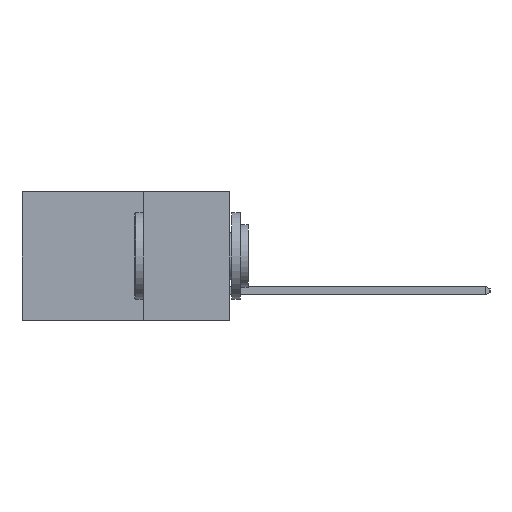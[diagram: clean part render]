
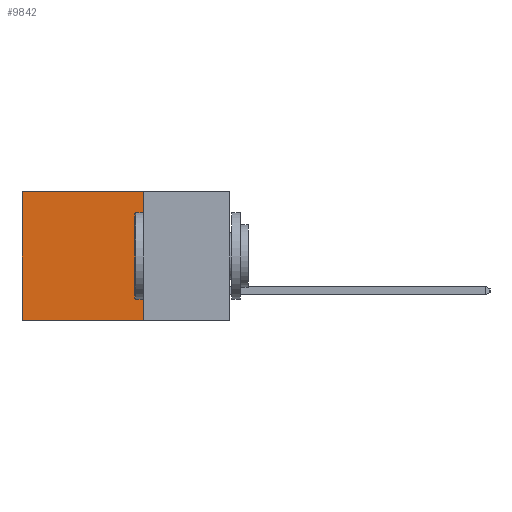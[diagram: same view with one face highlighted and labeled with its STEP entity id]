
A CAD part, left-side view. The second image highlights one B-rep face of the part: STEP entity #9842.
In plain terms, the highlighted planar face has unit normal (-1, 0, 0).
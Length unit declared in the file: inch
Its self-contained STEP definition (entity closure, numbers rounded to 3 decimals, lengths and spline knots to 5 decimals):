
#612 = EDGE_CURVE ( 'NONE', #9151, #3055, #3788, .T. ) ;
#982 = ORIENTED_EDGE ( 'NONE', *, *, #3374, .T. ) ;
#1239 = ORIENTED_EDGE ( 'NONE', *, *, #1735, .F. ) ;
#1649 = VECTOR ( 'NONE', #13019, 39.37008 ) ;
#1735 = EDGE_CURVE ( 'NONE', #12136, #3055, #7342, .T. ) ;
#2565 = CARTESIAN_POINT ( 'NONE',  ( 0.2615, 0.25, 0. ) ) ;
#3055 = VERTEX_POINT ( 'NONE', #4842 ) ;
#3374 = EDGE_CURVE ( 'NONE', #3661, #9151, #10922, .T. ) ;
#3661 = VERTEX_POINT ( 'NONE', #2565 ) ;
#3788 = LINE ( 'NONE', #11688, #6868 ) ;
#4416 = VECTOR ( 'NONE', #4444, 39.37008 ) ;
#4444 = DIRECTION ( 'NONE',  ( 0., 1., 0. ) ) ;
#4549 = VECTOR ( 'NONE', #10312, 39.37008 ) ;
#4842 = CARTESIAN_POINT ( 'NONE',  ( 0.2615, 0.6, -0.37 ) ) ;
#5397 = DIRECTION ( 'NONE',  ( 1., 0., 0. ) ) ;
#5766 = CARTESIAN_POINT ( 'NONE',  ( 0.2615, 0.25, -0.37 ) ) ;
#6208 = CARTESIAN_POINT ( 'NONE',  ( 0.2615, 0.25, -0.37 ) ) ;
#6597 = CARTESIAN_POINT ( 'NONE',  ( 0.2615, 0.25, -0.37 ) ) ;
#6868 = VECTOR ( 'NONE', #7545, 39.37008 ) ;
#7025 = CARTESIAN_POINT ( 'NONE',  ( 0.2615, 0.25, -0.37 ) ) ;
#7342 = LINE ( 'NONE', #6208, #4416 ) ;
#7545 = DIRECTION ( 'NONE',  ( 0., 0., -1. ) ) ;
#7558 = DIRECTION ( 'NONE',  ( 0., 0., -1. ) ) ;
#7623 = FACE_OUTER_BOUND ( 'NONE', #13405, .T. ) ;
#8495 = CARTESIAN_POINT ( 'NONE',  ( 0.2615, 0.25, 0. ) ) ;
#9014 = CARTESIAN_POINT ( 'NONE',  ( 0.2615, 0.6, 0. ) ) ;
#9151 = VERTEX_POINT ( 'NONE', #9014 ) ;
#9203 = EDGE_CURVE ( 'NONE', #3661, #12136, #9550, .T. ) ;
#9550 = LINE ( 'NONE', #5766, #4549 ) ;
#9842 = ADVANCED_FACE ( 'NONE', ( #7623 ), #11991, .F. ) ;
#10312 = DIRECTION ( 'NONE',  ( 0., 0., -1. ) ) ;
#10651 = AXIS2_PLACEMENT_3D ( 'NONE', #6597, #5397, #7558 ) ;
#10857 = ORIENTED_EDGE ( 'NONE', *, *, #612, .T. ) ;
#10922 = LINE ( 'NONE', #8495, #1649 ) ;
#11688 = CARTESIAN_POINT ( 'NONE',  ( 0.2615, 0.6, -0.37 ) ) ;
#11991 = PLANE ( 'NONE',  #10651 ) ;
#12136 = VERTEX_POINT ( 'NONE', #7025 ) ;
#13019 = DIRECTION ( 'NONE',  ( 0., 1., 0. ) ) ;
#13405 = EDGE_LOOP ( 'NONE', ( #10857, #1239, #14126, #982 ) ) ;
#14126 = ORIENTED_EDGE ( 'NONE', *, *, #9203, .F. ) ;
